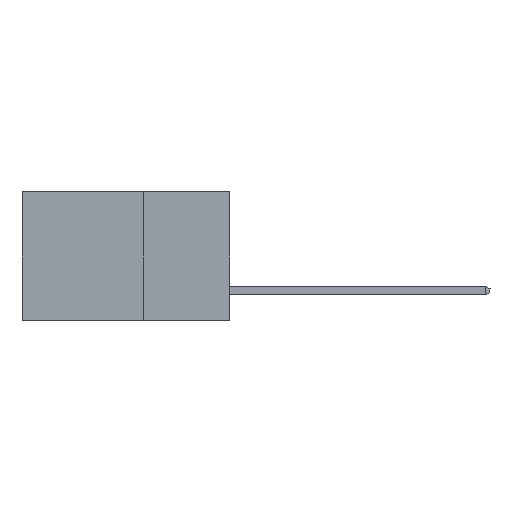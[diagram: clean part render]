
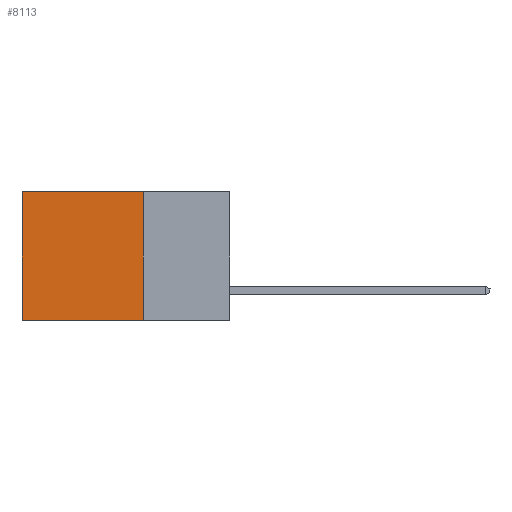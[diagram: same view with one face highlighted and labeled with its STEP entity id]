
A CAD part, left-side view. The second image highlights one B-rep face of the part: STEP entity #8113.
In plain terms, the highlighted planar face has unit normal (-1, 0, 0).
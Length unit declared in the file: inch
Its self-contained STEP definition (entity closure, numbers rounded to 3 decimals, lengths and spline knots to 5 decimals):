
#989 = VECTOR ( 'NONE', #10549, 39.37008 ) ;
#1138 = LINE ( 'NONE', #11392, #1676 ) ;
#1676 = VECTOR ( 'NONE', #10397, 39.37008 ) ;
#1869 = EDGE_CURVE ( 'NONE', #6341, #11538, #8168, .T. ) ;
#2168 = LINE ( 'NONE', #9748, #9114 ) ;
#2625 = VERTEX_POINT ( 'NONE', #5213 ) ;
#2627 = VERTEX_POINT ( 'NONE', #8985 ) ;
#2843 = CARTESIAN_POINT ( 'NONE',  ( 0.2615, 0.25, -0.37 ) ) ;
#2921 = CARTESIAN_POINT ( 'NONE',  ( 0.2615, 0.6, -0.37 ) ) ;
#2958 = FACE_OUTER_BOUND ( 'NONE', #10933, .T. ) ;
#3140 = VECTOR ( 'NONE', #7251, 39.37008 ) ;
#3409 = CARTESIAN_POINT ( 'NONE',  ( 0.2615, 0.6, -0.37 ) ) ;
#4570 = ORIENTED_EDGE ( 'NONE', *, *, #12000, .F. ) ;
#5053 = DIRECTION ( 'NONE',  ( 0., 1., 0. ) ) ;
#5213 = CARTESIAN_POINT ( 'NONE',  ( 0.2615, 0.25, -0.37 ) ) ;
#5223 = AXIS2_PLACEMENT_3D ( 'NONE', #11352, #5667, #9493 ) ;
#5667 = DIRECTION ( 'NONE',  ( 1., 0., 0. ) ) ;
#6341 = VERTEX_POINT ( 'NONE', #7799 ) ;
#6686 = EDGE_CURVE ( 'NONE', #2627, #6341, #2168, .T. ) ;
#7172 = ORIENTED_EDGE ( 'NONE', *, *, #1869, .T. ) ;
#7251 = DIRECTION ( 'NONE',  ( 0., 0., -1. ) ) ;
#7799 = CARTESIAN_POINT ( 'NONE',  ( 0.2615, 0.6, 0. ) ) ;
#7805 = ORIENTED_EDGE ( 'NONE', *, *, #8495, .F. ) ;
#8113 = ADVANCED_FACE ( 'NONE', ( #2958 ), #12216, .F. ) ;
#8168 = LINE ( 'NONE', #3409, #3140 ) ;
#8495 = EDGE_CURVE ( 'NONE', #2625, #11538, #1138, .T. ) ;
#8985 = CARTESIAN_POINT ( 'NONE',  ( 0.2615, 0.25, 0. ) ) ;
#9114 = VECTOR ( 'NONE', #5053, 39.37008 ) ;
#9493 = DIRECTION ( 'NONE',  ( 0., 0., -1. ) ) ;
#9666 = ORIENTED_EDGE ( 'NONE', *, *, #6686, .T. ) ;
#9748 = CARTESIAN_POINT ( 'NONE',  ( 0.2615, 0.25, 0. ) ) ;
#10397 = DIRECTION ( 'NONE',  ( 0., 1., 0. ) ) ;
#10549 = DIRECTION ( 'NONE',  ( 0., 0., -1. ) ) ;
#10933 = EDGE_LOOP ( 'NONE', ( #7172, #7805, #4570, #9666 ) ) ;
#11352 = CARTESIAN_POINT ( 'NONE',  ( 0.2615, 0.25, -0.37 ) ) ;
#11364 = LINE ( 'NONE', #2843, #989 ) ;
#11392 = CARTESIAN_POINT ( 'NONE',  ( 0.2615, 0.25, -0.37 ) ) ;
#11538 = VERTEX_POINT ( 'NONE', #2921 ) ;
#12000 = EDGE_CURVE ( 'NONE', #2627, #2625, #11364, .T. ) ;
#12216 = PLANE ( 'NONE',  #5223 ) ;
